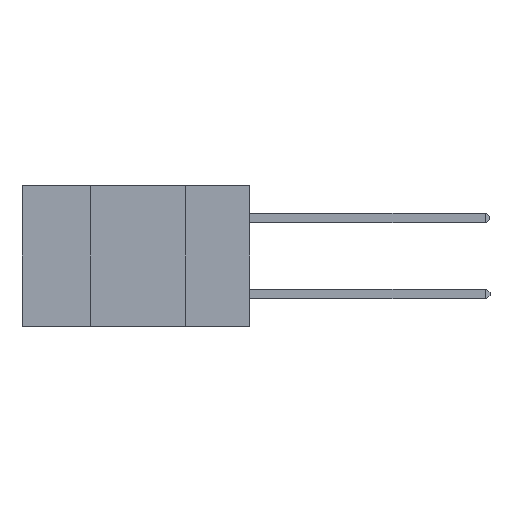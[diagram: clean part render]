
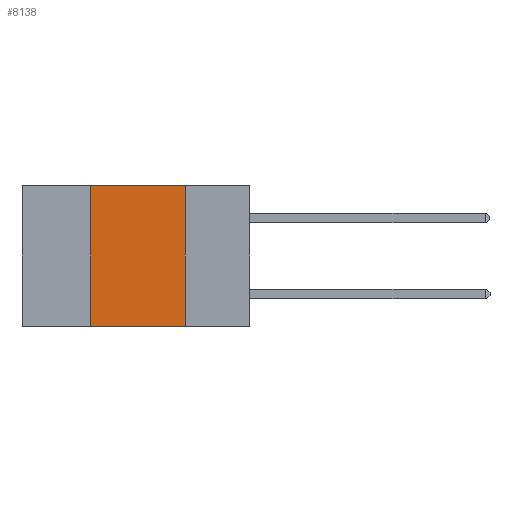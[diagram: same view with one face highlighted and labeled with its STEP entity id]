
A CAD part, left-side view. The second image highlights one B-rep face of the part: STEP entity #8138.
In plain terms, the highlighted planar face has unit normal (-1, 0, 0).
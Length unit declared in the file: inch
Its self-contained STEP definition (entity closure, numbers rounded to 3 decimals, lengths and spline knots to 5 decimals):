
#1231 = DIRECTION ( 'NONE',  ( 0., -1., 0. ) ) ;
#1291 = ORIENTED_EDGE ( 'NONE', *, *, #15426, .F. ) ;
#1629 = LINE ( 'NONE', #11090, #16019 ) ;
#2671 = DIRECTION ( 'NONE',  ( 0., 0., -1. ) ) ;
#2697 = CARTESIAN_POINT ( 'NONE',  ( 0., 0.17, -0.37 ) ) ;
#2823 = AXIS2_PLACEMENT_3D ( 'NONE', #9595, #11050, #2671 ) ;
#2922 = EDGE_LOOP ( 'NONE', ( #14656, #1291, #7553, #12021 ) ) ;
#4100 = EDGE_CURVE ( 'NONE', #11556, #16055, #17932, .T. ) ;
#5599 = CARTESIAN_POINT ( 'NONE',  ( 0., 0.42, 0. ) ) ;
#6032 = VECTOR ( 'NONE', #9099, 39.37008 ) ;
#6109 = DIRECTION ( 'NONE',  ( 0., -1., 0. ) ) ;
#6509 = EDGE_CURVE ( 'NONE', #8707, #16055, #13408, .T. ) ;
#6822 = VECTOR ( 'NONE', #6109, 39.37008 ) ;
#7553 = ORIENTED_EDGE ( 'NONE', *, *, #10289, .F. ) ;
#8138 = ADVANCED_FACE ( 'NONE', ( #11868 ), #12364, .F. ) ;
#8707 = VERTEX_POINT ( 'NONE', #9763 ) ;
#9099 = DIRECTION ( 'NONE',  ( 0., 0., -1. ) ) ;
#9595 = CARTESIAN_POINT ( 'NONE',  ( 0., 0.6, 0. ) ) ;
#9763 = CARTESIAN_POINT ( 'NONE',  ( 0., 0.17, 0. ) ) ;
#10277 = CARTESIAN_POINT ( 'NONE',  ( 0., 0.6, -0.37 ) ) ;
#10289 = EDGE_CURVE ( 'NONE', #11556, #15466, #13939, .T. ) ;
#11050 = DIRECTION ( 'NONE',  ( 1., 0., 0. ) ) ;
#11090 = CARTESIAN_POINT ( 'NONE',  ( 0., 0.6, 0. ) ) ;
#11556 = VERTEX_POINT ( 'NONE', #16545 ) ;
#11868 = FACE_OUTER_BOUND ( 'NONE', #2922, .T. ) ;
#12021 = ORIENTED_EDGE ( 'NONE', *, *, #4100, .T. ) ;
#12364 = PLANE ( 'NONE',  #2823 ) ;
#13408 = LINE ( 'NONE', #15961, #6032 ) ;
#13489 = VECTOR ( 'NONE', #16704, 39.37008 ) ;
#13939 = LINE ( 'NONE', #5599, #13489 ) ;
#14656 = ORIENTED_EDGE ( 'NONE', *, *, #6509, .F. ) ;
#15426 = EDGE_CURVE ( 'NONE', #15466, #8707, #1629, .T. ) ;
#15466 = VERTEX_POINT ( 'NONE', #18082 ) ;
#15961 = CARTESIAN_POINT ( 'NONE',  ( 0., 0.17, 0. ) ) ;
#16019 = VECTOR ( 'NONE', #1231, 39.37008 ) ;
#16055 = VERTEX_POINT ( 'NONE', #2697 ) ;
#16545 = CARTESIAN_POINT ( 'NONE',  ( 0., 0.42, -0.37 ) ) ;
#16704 = DIRECTION ( 'NONE',  ( 0., 0., 1. ) ) ;
#17932 = LINE ( 'NONE', #10277, #6822 ) ;
#18082 = CARTESIAN_POINT ( 'NONE',  ( 0., 0.42, 0. ) ) ;
